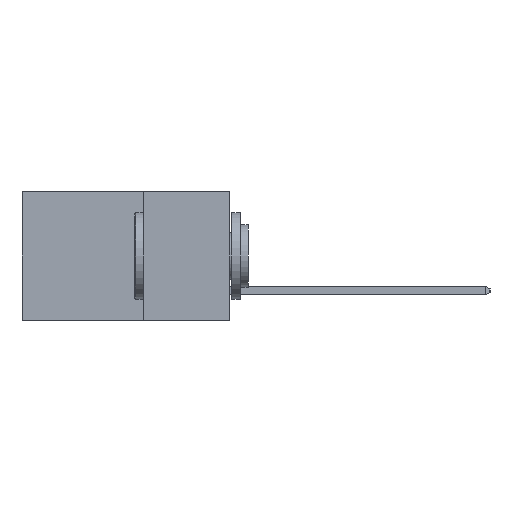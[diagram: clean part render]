
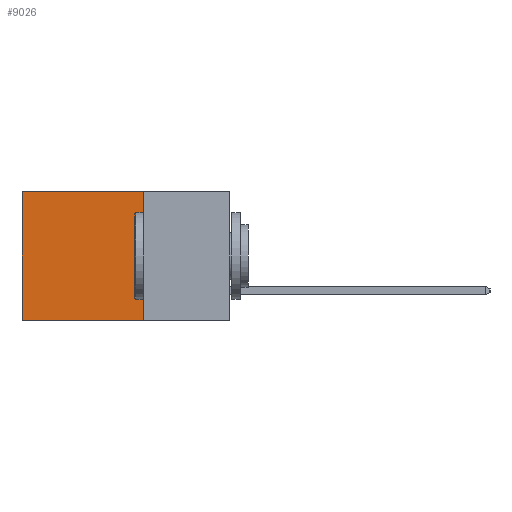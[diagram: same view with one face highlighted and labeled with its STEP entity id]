
A CAD part, left-side view. The second image highlights one B-rep face of the part: STEP entity #9026.
In plain terms, the highlighted planar face has unit normal (-1, 0, 0).
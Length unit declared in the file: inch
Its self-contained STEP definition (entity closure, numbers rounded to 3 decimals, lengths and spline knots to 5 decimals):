
#348 = CARTESIAN_POINT ( 'NONE',  ( 0.298, 0.25, 0. ) ) ;
#554 = DIRECTION ( 'NONE',  ( 0., 0., -1. ) ) ;
#2300 = CARTESIAN_POINT ( 'NONE',  ( 0.298, 0.25, -0.37 ) ) ;
#2408 = DIRECTION ( 'NONE',  ( 0., 0., -1. ) ) ;
#3243 = VECTOR ( 'NONE', #3399, 39.37008 ) ;
#3399 = DIRECTION ( 'NONE',  ( 0., 1., 0. ) ) ;
#3464 = VERTEX_POINT ( 'NONE', #5672 ) ;
#5354 = VECTOR ( 'NONE', #6893, 39.37008 ) ;
#5501 = FACE_OUTER_BOUND ( 'NONE', #13010, .T. ) ;
#5672 = CARTESIAN_POINT ( 'NONE',  ( 0.298, 0.25, 0. ) ) ;
#6463 = CARTESIAN_POINT ( 'NONE',  ( 0.298, 0.6, 0. ) ) ;
#6893 = DIRECTION ( 'NONE',  ( 0., 1., 0. ) ) ;
#7302 = LINE ( 'NONE', #348, #3243 ) ;
#7629 = LINE ( 'NONE', #13060, #15248 ) ;
#7682 = ORIENTED_EDGE ( 'NONE', *, *, #13539, .F. ) ;
#7777 = CARTESIAN_POINT ( 'NONE',  ( 0.298, 0.25, -0.37 ) ) ;
#7915 = VERTEX_POINT ( 'NONE', #6463 ) ;
#8096 = PLANE ( 'NONE',  #8946 ) ;
#8327 = CARTESIAN_POINT ( 'NONE',  ( 0.298, 0.6, -0.37 ) ) ;
#8946 = AXIS2_PLACEMENT_3D ( 'NONE', #18679, #9624, #554 ) ;
#9026 = ADVANCED_FACE ( 'NONE', ( #5501 ), #8096, .F. ) ;
#9624 = DIRECTION ( 'NONE',  ( 1., 0., 0. ) ) ;
#11540 = ORIENTED_EDGE ( 'NONE', *, *, #14455, .F. ) ;
#12217 = DIRECTION ( 'NONE',  ( 0., 0., -1. ) ) ;
#13010 = EDGE_LOOP ( 'NONE', ( #16324, #7682, #11540, #14941 ) ) ;
#13060 = CARTESIAN_POINT ( 'NONE',  ( 0.298, 0.6, 0. ) ) ;
#13431 = LINE ( 'NONE', #2300, #5354 ) ;
#13539 = EDGE_CURVE ( 'NONE', #18902, #15575, #13431, .T. ) ;
#14415 = LINE ( 'NONE', #15297, #18372 ) ;
#14455 = EDGE_CURVE ( 'NONE', #3464, #18902, #14415, .T. ) ;
#14941 = ORIENTED_EDGE ( 'NONE', *, *, #16917, .T. ) ;
#15248 = VECTOR ( 'NONE', #2408, 39.37008 ) ;
#15297 = CARTESIAN_POINT ( 'NONE',  ( 0.298, 0.25, 0. ) ) ;
#15575 = VERTEX_POINT ( 'NONE', #8327 ) ;
#16324 = ORIENTED_EDGE ( 'NONE', *, *, #16518, .T. ) ;
#16518 = EDGE_CURVE ( 'NONE', #7915, #15575, #7629, .T. ) ;
#16917 = EDGE_CURVE ( 'NONE', #3464, #7915, #7302, .T. ) ;
#18372 = VECTOR ( 'NONE', #12217, 39.37008 ) ;
#18679 = CARTESIAN_POINT ( 'NONE',  ( 0.298, 0.25, 0. ) ) ;
#18902 = VERTEX_POINT ( 'NONE', #7777 ) ;
